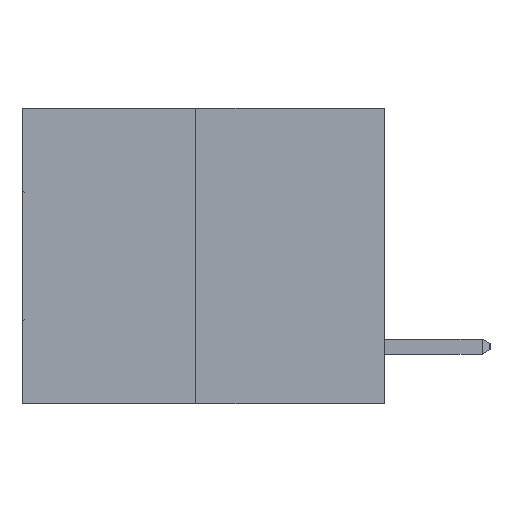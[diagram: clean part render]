
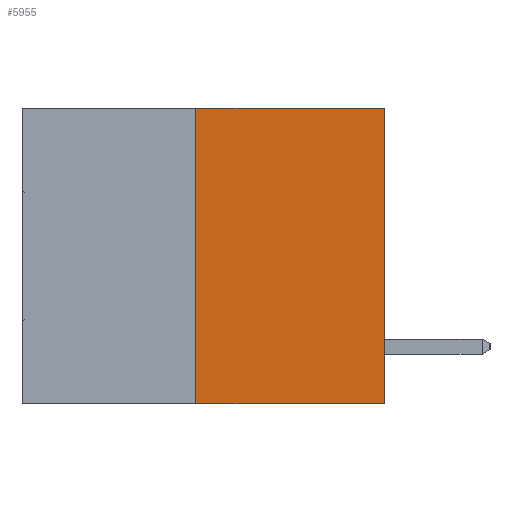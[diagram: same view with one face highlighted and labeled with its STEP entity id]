
A CAD part, left-side view. The second image highlights one B-rep face of the part: STEP entity #5955.
In plain terms, the highlighted planar face has unit normal (-1, 0, 0).
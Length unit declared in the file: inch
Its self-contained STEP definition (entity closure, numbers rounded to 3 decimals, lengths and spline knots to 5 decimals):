
#124 = EDGE_CURVE ( 'NONE', #33457, #22562, #30400, .T. ) ;
#725 = VECTOR ( 'NONE', #6325, 39.37008 ) ;
#1510 = LINE ( 'NONE', #21754, #14926 ) ;
#2846 = ORIENTED_EDGE ( 'NONE', *, *, #13401, .F. ) ;
#4935 = LINE ( 'NONE', #20229, #10631 ) ;
#5955 = ADVANCED_FACE ( 'NONE', ( #6678 ), #13587, .F. ) ;
#6070 = CARTESIAN_POINT ( 'NONE',  ( 0., 0.312, 0. ) ) ;
#6108 = DIRECTION ( 'NONE',  ( 0., -1., 0. ) ) ;
#6325 = DIRECTION ( 'NONE',  ( 0., -1., 0. ) ) ;
#6678 = FACE_OUTER_BOUND ( 'NONE', #10646, .T. ) ;
#7099 = ORIENTED_EDGE ( 'NONE', *, *, #29629, .F. ) ;
#7861 = VERTEX_POINT ( 'NONE', #6070 ) ;
#8472 = DIRECTION ( 'NONE',  ( 1., 0., 0. ) ) ;
#8797 = CARTESIAN_POINT ( 'NONE',  ( 0., 0., 0. ) ) ;
#8943 = CARTESIAN_POINT ( 'NONE',  ( 0., 0.6, 0. ) ) ;
#10458 = VECTOR ( 'NONE', #6108, 39.37008 ) ;
#10631 = VECTOR ( 'NONE', #27019, 39.37008 ) ;
#10646 = EDGE_LOOP ( 'NONE', ( #2846, #16284, #26390, #7099 ) ) ;
#13401 = EDGE_CURVE ( 'NONE', #33457, #7861, #1510, .T. ) ;
#13587 = PLANE ( 'NONE',  #14689 ) ;
#14689 = AXIS2_PLACEMENT_3D ( 'NONE', #24088, #8472, #16228 ) ;
#14926 = VECTOR ( 'NONE', #29175, 39.37008 ) ;
#15603 = CARTESIAN_POINT ( 'NONE',  ( 0., 0.312, -0.49 ) ) ;
#16228 = DIRECTION ( 'NONE',  ( 0., 0., -1. ) ) ;
#16284 = ORIENTED_EDGE ( 'NONE', *, *, #124, .T. ) ;
#17394 = LINE ( 'NONE', #8943, #10458 ) ;
#20229 = CARTESIAN_POINT ( 'NONE',  ( 0., 0., 0. ) ) ;
#20395 = EDGE_CURVE ( 'NONE', #22562, #22049, #4935, .T. ) ;
#21754 = CARTESIAN_POINT ( 'NONE',  ( 0., 0.312, -0.49 ) ) ;
#22049 = VERTEX_POINT ( 'NONE', #8797 ) ;
#22562 = VERTEX_POINT ( 'NONE', #32508 ) ;
#24088 = CARTESIAN_POINT ( 'NONE',  ( 0., 0.6, 0. ) ) ;
#26390 = ORIENTED_EDGE ( 'NONE', *, *, #20395, .T. ) ;
#26939 = CARTESIAN_POINT ( 'NONE',  ( 0., 0.6, -0.49 ) ) ;
#27019 = DIRECTION ( 'NONE',  ( 0., 0., 1. ) ) ;
#29175 = DIRECTION ( 'NONE',  ( 0., 0., 1. ) ) ;
#29629 = EDGE_CURVE ( 'NONE', #7861, #22049, #17394, .T. ) ;
#30400 = LINE ( 'NONE', #26939, #725 ) ;
#32508 = CARTESIAN_POINT ( 'NONE',  ( 0., 0., -0.49 ) ) ;
#33457 = VERTEX_POINT ( 'NONE', #15603 ) ;
